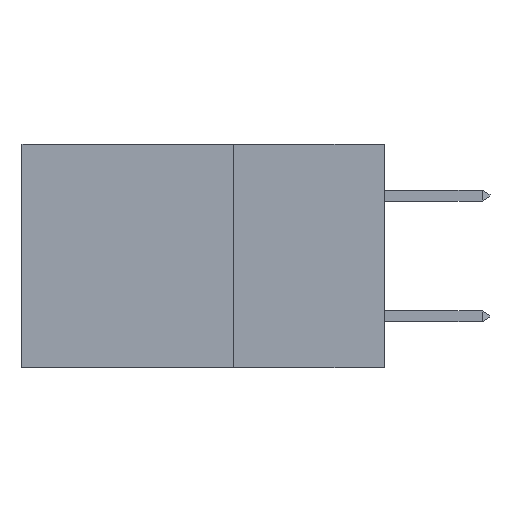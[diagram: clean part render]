
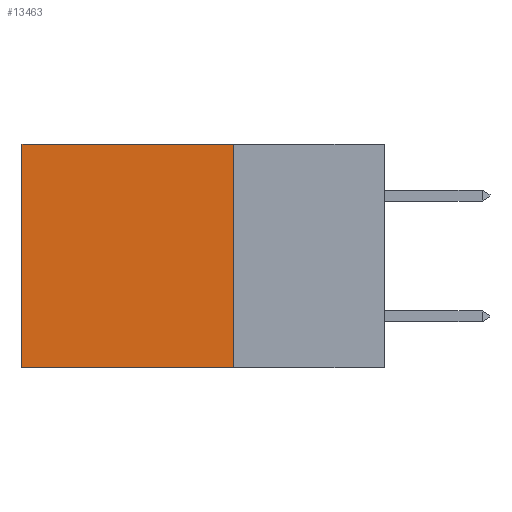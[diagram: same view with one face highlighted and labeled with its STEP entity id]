
A CAD part, left-side view. The second image highlights one B-rep face of the part: STEP entity #13463.
In plain terms, the highlighted planar face has unit normal (-1, 0, 0).
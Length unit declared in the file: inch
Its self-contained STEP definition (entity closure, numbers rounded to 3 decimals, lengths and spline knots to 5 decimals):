
#152 = EDGE_CURVE ( 'NONE', #11716, #4106, #14045, .T. ) ;
#450 = DIRECTION ( 'NONE',  ( 0., 0., -1. ) ) ;
#1179 = CARTESIAN_POINT ( 'NONE',  ( 0.2875, 0.6, 0. ) ) ;
#1904 = EDGE_LOOP ( 'NONE', ( #9970, #3766, #12335, #3148 ) ) ;
#2739 = FACE_OUTER_BOUND ( 'NONE', #1904, .T. ) ;
#2788 = CARTESIAN_POINT ( 'NONE',  ( 0.2875, 0.25, -0.37 ) ) ;
#2794 = CARTESIAN_POINT ( 'NONE',  ( 0.2875, 0.25, 0. ) ) ;
#3148 = ORIENTED_EDGE ( 'NONE', *, *, #12158, .T. ) ;
#3539 = VECTOR ( 'NONE', #7417, 39.37008 ) ;
#3544 = DIRECTION ( 'NONE',  ( 0., 0., -1. ) ) ;
#3766 = ORIENTED_EDGE ( 'NONE', *, *, #9901, .F. ) ;
#3777 = VECTOR ( 'NONE', #10860, 39.37008 ) ;
#3802 = VERTEX_POINT ( 'NONE', #13525 ) ;
#4065 = DIRECTION ( 'NONE',  ( 0., 0., -1. ) ) ;
#4106 = VERTEX_POINT ( 'NONE', #5213 ) ;
#4458 = AXIS2_PLACEMENT_3D ( 'NONE', #13205, #7591, #450 ) ;
#4843 = CARTESIAN_POINT ( 'NONE',  ( 0.2875, 0.6, 0. ) ) ;
#5213 = CARTESIAN_POINT ( 'NONE',  ( 0.2875, 0.6, -0.37 ) ) ;
#6528 = LINE ( 'NONE', #2794, #3539 ) ;
#7417 = DIRECTION ( 'NONE',  ( 0., 1., 0. ) ) ;
#7591 = DIRECTION ( 'NONE',  ( 1., 0., 0. ) ) ;
#9901 = EDGE_CURVE ( 'NONE', #10279, #4106, #12505, .T. ) ;
#9970 = ORIENTED_EDGE ( 'NONE', *, *, #152, .T. ) ;
#10279 = VERTEX_POINT ( 'NONE', #13727 ) ;
#10854 = VECTOR ( 'NONE', #3544, 39.37008 ) ;
#10860 = DIRECTION ( 'NONE',  ( 0., 1., 0. ) ) ;
#11716 = VERTEX_POINT ( 'NONE', #4843 ) ;
#12096 = LINE ( 'NONE', #13125, #14873 ) ;
#12127 = PLANE ( 'NONE',  #4458 ) ;
#12158 = EDGE_CURVE ( 'NONE', #3802, #11716, #6528, .T. ) ;
#12335 = ORIENTED_EDGE ( 'NONE', *, *, #12839, .F. ) ;
#12505 = LINE ( 'NONE', #2788, #3777 ) ;
#12839 = EDGE_CURVE ( 'NONE', #3802, #10279, #12096, .T. ) ;
#13125 = CARTESIAN_POINT ( 'NONE',  ( 0.2875, 0.25, 0. ) ) ;
#13205 = CARTESIAN_POINT ( 'NONE',  ( 0.2875, 0.25, 0. ) ) ;
#13463 = ADVANCED_FACE ( 'NONE', ( #2739 ), #12127, .F. ) ;
#13525 = CARTESIAN_POINT ( 'NONE',  ( 0.2875, 0.25, 0. ) ) ;
#13727 = CARTESIAN_POINT ( 'NONE',  ( 0.2875, 0.25, -0.37 ) ) ;
#14045 = LINE ( 'NONE', #1179, #10854 ) ;
#14873 = VECTOR ( 'NONE', #4065, 39.37008 ) ;
